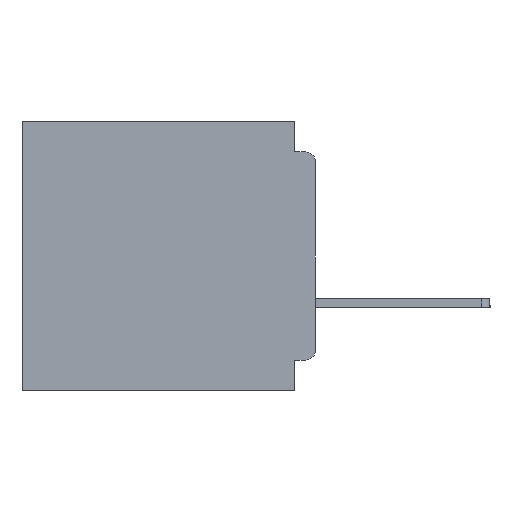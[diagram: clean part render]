
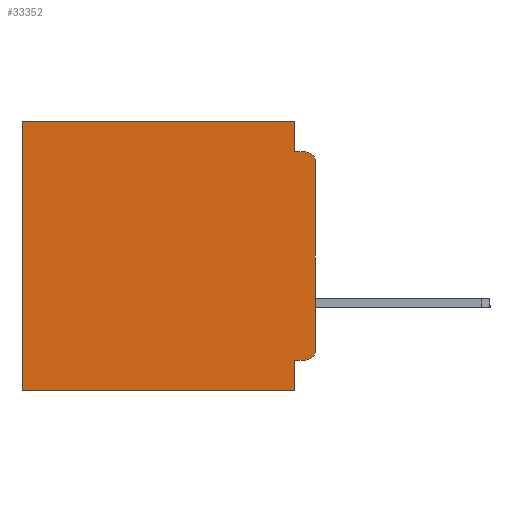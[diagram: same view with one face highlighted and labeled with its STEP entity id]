
A CAD part, left-side view. The second image highlights one B-rep face of the part: STEP entity #33352.
In plain terms, the highlighted planar face has unit normal (-1, 0, 0).
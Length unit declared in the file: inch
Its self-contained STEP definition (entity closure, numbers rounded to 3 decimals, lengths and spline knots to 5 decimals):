
#757 = CIRCLE ( 'NONE', #12734, 0.015 ) ;
#1094 = DIRECTION ( 'NONE',  ( -1., 0., 0. ) ) ;
#1737 = VERTEX_POINT ( 'NONE', #20896 ) ;
#2330 = CARTESIAN_POINT ( 'NONE',  ( 0.3, 0.031, -0.355 ) ) ;
#3259 = VECTOR ( 'NONE', #32600, 39.37008 ) ;
#3898 = VECTOR ( 'NONE', #24787, 39.37008 ) ;
#4619 = DIRECTION ( 'NONE',  ( 0., -1., 0. ) ) ;
#4947 = ORIENTED_EDGE ( 'NONE', *, *, #16463, .T. ) ;
#5331 = VECTOR ( 'NONE', #6708, 39.37008 ) ;
#6087 = CARTESIAN_POINT ( 'NONE',  ( 0.3, 0., -0.34 ) ) ;
#6127 = ORIENTED_EDGE ( 'NONE', *, *, #35816, .T. ) ;
#6255 = ORIENTED_EDGE ( 'NONE', *, *, #20702, .F. ) ;
#6422 = LINE ( 'NONE', #6861, #5331 ) ;
#6708 = DIRECTION ( 'NONE',  ( 0., 1., 0. ) ) ;
#6793 = EDGE_CURVE ( 'NONE', #21068, #16792, #33397, .T. ) ;
#6820 = DIRECTION ( 'NONE',  ( 0., 0., -1. ) ) ;
#6861 = CARTESIAN_POINT ( 'NONE',  ( 0.3, 0., 0. ) ) ;
#8298 = ORIENTED_EDGE ( 'NONE', *, *, #42617, .F. ) ;
#9477 = ORIENTED_EDGE ( 'NONE', *, *, #10596, .F. ) ;
#10244 = EDGE_LOOP ( 'NONE', ( #8298, #43727, #25996, #6255, #43607, #6127, #9477, #29497, #29696, #4947 ) ) ;
#10499 = DIRECTION ( 'NONE',  ( 0., 1., 0. ) ) ;
#10596 = EDGE_CURVE ( 'NONE', #16792, #32874, #30768, .T. ) ;
#10799 = VECTOR ( 'NONE', #6820, 39.37008 ) ;
#11993 = VECTOR ( 'NONE', #4619, 39.37008 ) ;
#12734 = AXIS2_PLACEMENT_3D ( 'NONE', #18813, #43032, #22308 ) ;
#12828 = CARTESIAN_POINT ( 'NONE',  ( 0.3, 0.031, -0.045 ) ) ;
#14281 = LINE ( 'NONE', #38645, #3898 ) ;
#14853 = LINE ( 'NONE', #17753, #32276 ) ;
#14881 = VECTOR ( 'NONE', #26378, 39.37008 ) ;
#15410 = VERTEX_POINT ( 'NONE', #43521 ) ;
#15850 = DIRECTION ( 'NONE',  ( 0., 0., -1. ) ) ;
#16463 = EDGE_CURVE ( 'NONE', #20077, #18970, #22820, .T. ) ;
#16792 = VERTEX_POINT ( 'NONE', #30656 ) ;
#16930 = VERTEX_POINT ( 'NONE', #31568 ) ;
#17068 = EDGE_CURVE ( 'NONE', #28380, #31982, #21133, .T. ) ;
#17753 = CARTESIAN_POINT ( 'NONE',  ( 0.3, 0.031, 0. ) ) ;
#17787 = LINE ( 'NONE', #41527, #10799 ) ;
#18376 = AXIS2_PLACEMENT_3D ( 'NONE', #21954, #1094, #25466 ) ;
#18436 = CARTESIAN_POINT ( 'NONE',  ( 0.3, 0., -0.045 ) ) ;
#18540 = CARTESIAN_POINT ( 'NONE',  ( 0.3, 0.437, -0.4 ) ) ;
#18813 = CARTESIAN_POINT ( 'NONE',  ( 0.3, 0.015, -0.06 ) ) ;
#18970 = VERTEX_POINT ( 'NONE', #6087 ) ;
#20077 = VERTEX_POINT ( 'NONE', #23588 ) ;
#20275 = EDGE_CURVE ( 'NONE', #20077, #21068, #14281, .T. ) ;
#20702 = EDGE_CURVE ( 'NONE', #15410, #28380, #14853, .T. ) ;
#20896 = CARTESIAN_POINT ( 'NONE',  ( 0.3, 0., -0.06 ) ) ;
#21068 = VERTEX_POINT ( 'NONE', #2330 ) ;
#21133 = LINE ( 'NONE', #18436, #11993 ) ;
#21229 = DIRECTION ( 'NONE',  ( 0., 0., -1. ) ) ;
#21459 = VECTOR ( 'NONE', #10499, 39.37008 ) ;
#21954 = CARTESIAN_POINT ( 'NONE',  ( 0.3, 0.015, -0.34 ) ) ;
#22308 = DIRECTION ( 'NONE',  ( 0., 0., -1. ) ) ;
#22820 = CIRCLE ( 'NONE', #18376, 0.015 ) ;
#23588 = CARTESIAN_POINT ( 'NONE',  ( 0.3, 0.015, -0.355 ) ) ;
#23619 = CARTESIAN_POINT ( 'NONE',  ( 0.3, 0.437, -0.4 ) ) ;
#24787 = DIRECTION ( 'NONE',  ( 0., 1., 0. ) ) ;
#25466 = DIRECTION ( 'NONE',  ( 0., 0., -1. ) ) ;
#25902 = FACE_OUTER_BOUND ( 'NONE', #10244, .T. ) ;
#25996 = ORIENTED_EDGE ( 'NONE', *, *, #17068, .F. ) ;
#26378 = DIRECTION ( 'NONE',  ( 0., 0., -1. ) ) ;
#27041 = CARTESIAN_POINT ( 'NONE',  ( 0.3, 0.031, -0.4 ) ) ;
#28380 = VERTEX_POINT ( 'NONE', #12828 ) ;
#29497 = ORIENTED_EDGE ( 'NONE', *, *, #6793, .F. ) ;
#29529 = CARTESIAN_POINT ( 'NONE',  ( 0.3, 0.015, -0.045 ) ) ;
#29696 = ORIENTED_EDGE ( 'NONE', *, *, #20275, .F. ) ;
#30656 = CARTESIAN_POINT ( 'NONE',  ( 0.3, 0.031, -0.4 ) ) ;
#30768 = LINE ( 'NONE', #31298, #21459 ) ;
#31052 = LINE ( 'NONE', #18540, #3259 ) ;
#31298 = CARTESIAN_POINT ( 'NONE',  ( 0.3, 0., -0.4 ) ) ;
#31568 = CARTESIAN_POINT ( 'NONE',  ( 0.3, 0.437, 0. ) ) ;
#31982 = VERTEX_POINT ( 'NONE', #29529 ) ;
#32276 = VECTOR ( 'NONE', #21229, 39.37008 ) ;
#32322 = EDGE_CURVE ( 'NONE', #15410, #16930, #6422, .T. ) ;
#32600 = DIRECTION ( 'NONE',  ( 0., 0., -1. ) ) ;
#32874 = VERTEX_POINT ( 'NONE', #23619 ) ;
#33084 = CARTESIAN_POINT ( 'NONE',  ( 0.3, 0., -0.4 ) ) ;
#33226 = PLANE ( 'NONE',  #33412 ) ;
#33352 = ADVANCED_FACE ( 'NONE', ( #25902 ), #33226, .F. ) ;
#33397 = LINE ( 'NONE', #27041, #14881 ) ;
#33412 = AXIS2_PLACEMENT_3D ( 'NONE', #33084, #36695, #15850 ) ;
#35816 = EDGE_CURVE ( 'NONE', #16930, #32874, #31052, .T. ) ;
#36695 = DIRECTION ( 'NONE',  ( 1., 0., 0. ) ) ;
#38645 = CARTESIAN_POINT ( 'NONE',  ( 0.3, 0., -0.355 ) ) ;
#41527 = CARTESIAN_POINT ( 'NONE',  ( 0.3, 0., -0.4 ) ) ;
#42617 = EDGE_CURVE ( 'NONE', #1737, #18970, #17787, .T. ) ;
#43032 = DIRECTION ( 'NONE',  ( -1., 0., 0. ) ) ;
#43521 = CARTESIAN_POINT ( 'NONE',  ( 0.3, 0.031, 0. ) ) ;
#43607 = ORIENTED_EDGE ( 'NONE', *, *, #32322, .T. ) ;
#43727 = ORIENTED_EDGE ( 'NONE', *, *, #44277, .T. ) ;
#44277 = EDGE_CURVE ( 'NONE', #1737, #31982, #757, .T. ) ;
